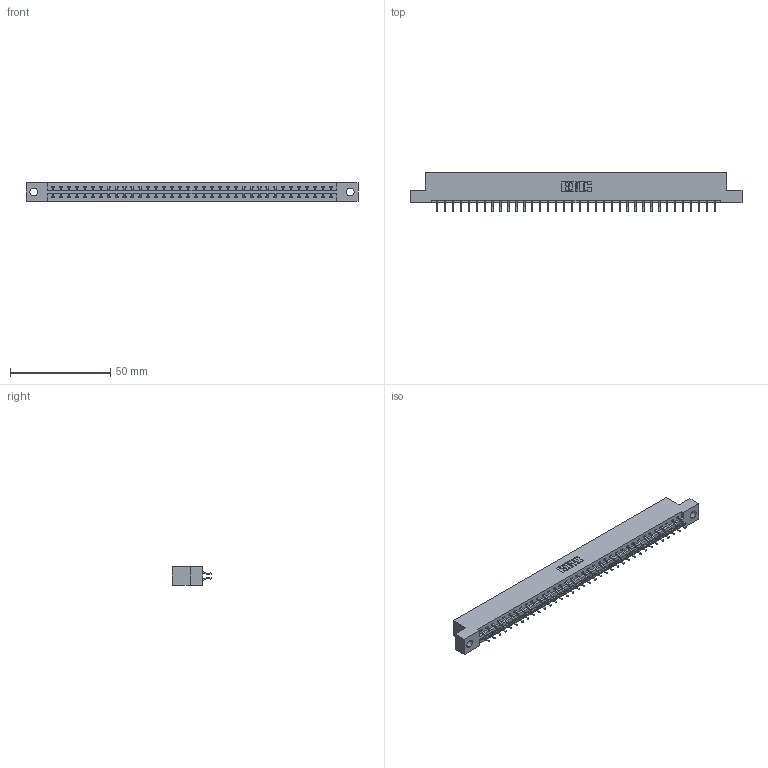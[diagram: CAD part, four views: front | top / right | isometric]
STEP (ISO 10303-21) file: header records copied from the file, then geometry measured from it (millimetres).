
FILE_DESCRIPTION (( 'STEP AP203' ), '1' );
FILE_NAME ('337-072-556-204.STEP', '2018-08-11T15:30:14', ( '' ), ( '' ), 'SwSTEP 2.0', 'SolidWorks 2016', '' );
FILE_SCHEMA (( 'CONFIG_CONTROL_DESIGN' ));
Length unit declared in the file: inch
Products named in the file (3): 337 Part_Flush Mounting Lugs - 0.156 Dia-TH; 345-292-001_556 Tail; 337-072-556-204
Assembly tree (73 placements, depth 2):
  337-072-556-204
    337 Part_Flush Mounting Lugs - 0.156 Dia-TH
    345-292-001_556 Tail  x72
Bounding box: 165.66 x 19.57 x 9.4 mm (x, y, z)
Volume: 17287.9 mm3; surface area: 19207.1 mm2
Topology: 73 solids, 73 shells, 4434 faces, 13199 edges, 8702 vertices
Faces by surface type: plane 3094, cylinder 1340
Entity records: 28911 total; most frequent: CARTESIAN_POINT 4890, ORIENTED_EDGE 4814, DIRECTION 4159, EDGE_CURVE 2407, VECTOR 2271, LINE 2271, VERTEX_POINT 1602, AXIS2_PLACEMENT_3D 944
